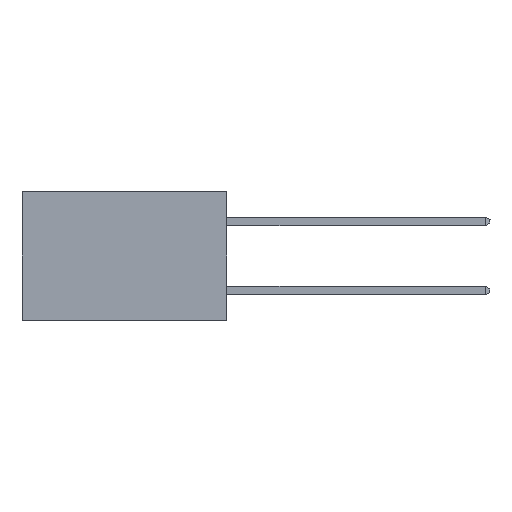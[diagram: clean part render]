
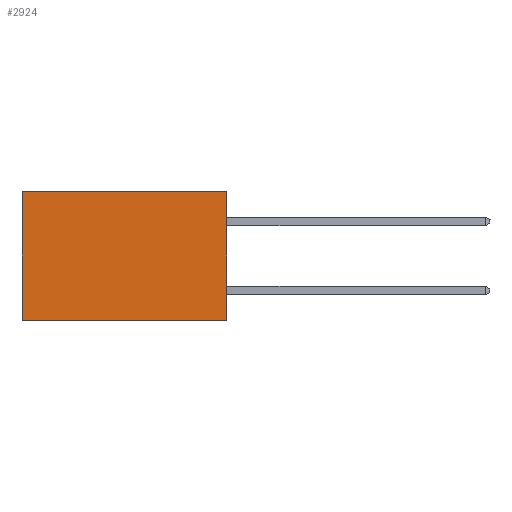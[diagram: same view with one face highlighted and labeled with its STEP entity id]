
A CAD part, left-side view. The second image highlights one B-rep face of the part: STEP entity #2924.
In plain terms, the highlighted planar face has unit normal (-1, 0, 0).
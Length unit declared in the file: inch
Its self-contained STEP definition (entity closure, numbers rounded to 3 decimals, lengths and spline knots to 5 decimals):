
#147 = VERTEX_POINT ( 'NONE', #8315 ) ;
#252 = CARTESIAN_POINT ( 'NONE',  ( 0.277, 0., -0.37 ) ) ;
#350 = LINE ( 'NONE', #484, #3898 ) ;
#454 = DIRECTION ( 'NONE',  ( 0., 1., 0. ) ) ;
#484 = CARTESIAN_POINT ( 'NONE',  ( 0.277, 0., 0. ) ) ;
#571 = LINE ( 'NONE', #5664, #3883 ) ;
#1629 = ORIENTED_EDGE ( 'NONE', *, *, #5150, .T. ) ;
#2449 = ORIENTED_EDGE ( 'NONE', *, *, #3842, .F. ) ;
#2516 = VERTEX_POINT ( 'NONE', #3267 ) ;
#2717 = VERTEX_POINT ( 'NONE', #252 ) ;
#2763 = ORIENTED_EDGE ( 'NONE', *, *, #6185, .T. ) ;
#2820 = EDGE_LOOP ( 'NONE', ( #2763, #7482, #2449, #1629 ) ) ;
#2869 = AXIS2_PLACEMENT_3D ( 'NONE', #6142, #6049, #6040 ) ;
#2892 = DIRECTION ( 'NONE',  ( 0., 0., -1. ) ) ;
#2900 = LINE ( 'NONE', #8118, #4340 ) ;
#2924 = ADVANCED_FACE ( 'NONE', ( #6827 ), #6059, .F. ) ;
#3267 = CARTESIAN_POINT ( 'NONE',  ( 0.277, 0.59, -0.37 ) ) ;
#3729 = LINE ( 'NONE', #4543, #8277 ) ;
#3842 = EDGE_CURVE ( 'NONE', #147, #2717, #3729, .T. ) ;
#3883 = VECTOR ( 'NONE', #5701, 39.37008 ) ;
#3898 = VECTOR ( 'NONE', #454, 39.37008 ) ;
#4288 = CARTESIAN_POINT ( 'NONE',  ( 0.277, 0.59, 0. ) ) ;
#4340 = VECTOR ( 'NONE', #8027, 39.37008 ) ;
#4543 = CARTESIAN_POINT ( 'NONE',  ( 0.277, 0., -0.37 ) ) ;
#4718 = VERTEX_POINT ( 'NONE', #4288 ) ;
#5150 = EDGE_CURVE ( 'NONE', #147, #4718, #350, .T. ) ;
#5664 = CARTESIAN_POINT ( 'NONE',  ( 0.277, 0.59, -0.37 ) ) ;
#5701 = DIRECTION ( 'NONE',  ( 0., 0., -1. ) ) ;
#5840 = EDGE_CURVE ( 'NONE', #2717, #2516, #2900, .T. ) ;
#6040 = DIRECTION ( 'NONE',  ( 0., 0., -1. ) ) ;
#6049 = DIRECTION ( 'NONE',  ( 1., 0., 0. ) ) ;
#6059 = PLANE ( 'NONE',  #2869 ) ;
#6142 = CARTESIAN_POINT ( 'NONE',  ( 0.277, 0., -0.37 ) ) ;
#6185 = EDGE_CURVE ( 'NONE', #4718, #2516, #571, .T. ) ;
#6827 = FACE_OUTER_BOUND ( 'NONE', #2820, .T. ) ;
#7482 = ORIENTED_EDGE ( 'NONE', *, *, #5840, .F. ) ;
#8027 = DIRECTION ( 'NONE',  ( 0., 1., 0. ) ) ;
#8118 = CARTESIAN_POINT ( 'NONE',  ( 0.277, 0., -0.37 ) ) ;
#8277 = VECTOR ( 'NONE', #2892, 39.37008 ) ;
#8315 = CARTESIAN_POINT ( 'NONE',  ( 0.277, 0., 0. ) ) ;
